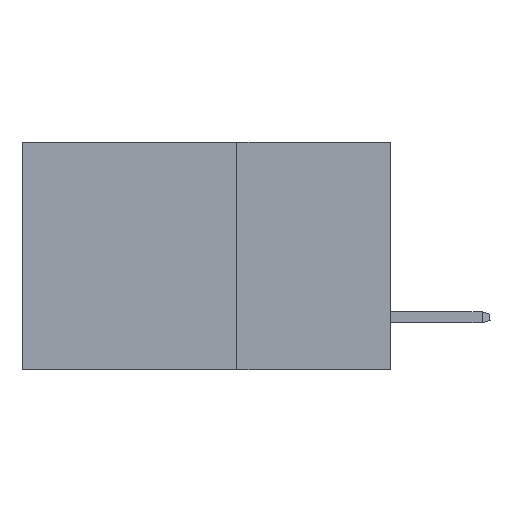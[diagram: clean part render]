
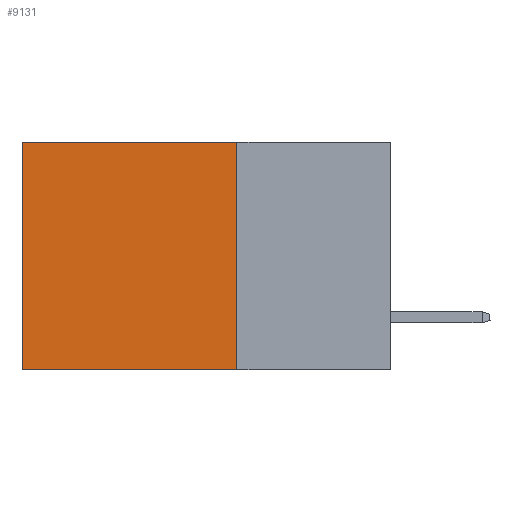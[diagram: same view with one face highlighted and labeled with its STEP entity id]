
A CAD part, left-side view. The second image highlights one B-rep face of the part: STEP entity #9131.
In plain terms, the highlighted planar face has unit normal (-1, 0, 0).
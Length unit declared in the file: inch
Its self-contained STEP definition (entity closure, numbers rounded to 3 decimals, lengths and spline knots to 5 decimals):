
#2479 = ORIENTED_EDGE ( 'NONE', *, *, #14598, .T. ) ;
#3785 = CARTESIAN_POINT ( 'NONE',  ( 0.2875, 0.25, -0.37 ) ) ;
#3862 = CARTESIAN_POINT ( 'NONE',  ( 0.2875, 0.25, 0. ) ) ;
#3996 = DIRECTION ( 'NONE',  ( 1., 0., 0. ) ) ;
#4401 = CARTESIAN_POINT ( 'NONE',  ( 0.2875, 0.25, 0. ) ) ;
#4408 = CARTESIAN_POINT ( 'NONE',  ( 0.2875, 0.25, 0. ) ) ;
#4504 = LINE ( 'NONE', #33628, #34681 ) ;
#5905 = EDGE_CURVE ( 'NONE', #17264, #22292, #32644, .T. ) ;
#6811 = DIRECTION ( 'NONE',  ( 0., 0., -1. ) ) ;
#7809 = EDGE_CURVE ( 'NONE', #28607, #22292, #4504, .T. ) ;
#8495 = CARTESIAN_POINT ( 'NONE',  ( 0.2875, 0.6, -0.37 ) ) ;
#9131 = ADVANCED_FACE ( 'NONE', ( #20010 ), #32714, .F. ) ;
#12883 = LINE ( 'NONE', #4401, #33358 ) ;
#13272 = DIRECTION ( 'NONE',  ( 0., 1., 0. ) ) ;
#14228 = VECTOR ( 'NONE', #13272, 39.37008 ) ;
#14277 = DIRECTION ( 'NONE',  ( 0., 1., 0. ) ) ;
#14598 = EDGE_CURVE ( 'NONE', #28910, #28607, #29687, .T. ) ;
#15638 = ORIENTED_EDGE ( 'NONE', *, *, #7809, .T. ) ;
#16763 = EDGE_LOOP ( 'NONE', ( #15638, #36933, #27501, #2479 ) ) ;
#17264 = VERTEX_POINT ( 'NONE', #3785 ) ;
#19887 = CARTESIAN_POINT ( 'NONE',  ( 0.2875, 0.25, -0.37 ) ) ;
#20010 = FACE_OUTER_BOUND ( 'NONE', #16763, .T. ) ;
#22292 = VERTEX_POINT ( 'NONE', #8495 ) ;
#24111 = CARTESIAN_POINT ( 'NONE',  ( 0.2875, 0.6, 0. ) ) ;
#27501 = ORIENTED_EDGE ( 'NONE', *, *, #37547, .F. ) ;
#28607 = VERTEX_POINT ( 'NONE', #24111 ) ;
#28910 = VERTEX_POINT ( 'NONE', #32113 ) ;
#29687 = LINE ( 'NONE', #4408, #14228 ) ;
#30806 = DIRECTION ( 'NONE',  ( 0., 0., -1. ) ) ;
#31209 = AXIS2_PLACEMENT_3D ( 'NONE', #3862, #3996, #6811 ) ;
#32113 = CARTESIAN_POINT ( 'NONE',  ( 0.2875, 0.25, 0. ) ) ;
#32233 = VECTOR ( 'NONE', #14277, 39.37008 ) ;
#32644 = LINE ( 'NONE', #19887, #32233 ) ;
#32714 = PLANE ( 'NONE',  #31209 ) ;
#33358 = VECTOR ( 'NONE', #33630, 39.37008 ) ;
#33628 = CARTESIAN_POINT ( 'NONE',  ( 0.2875, 0.6, 0. ) ) ;
#33630 = DIRECTION ( 'NONE',  ( 0., 0., -1. ) ) ;
#34681 = VECTOR ( 'NONE', #30806, 39.37008 ) ;
#36933 = ORIENTED_EDGE ( 'NONE', *, *, #5905, .F. ) ;
#37547 = EDGE_CURVE ( 'NONE', #28910, #17264, #12883, .T. ) ;
